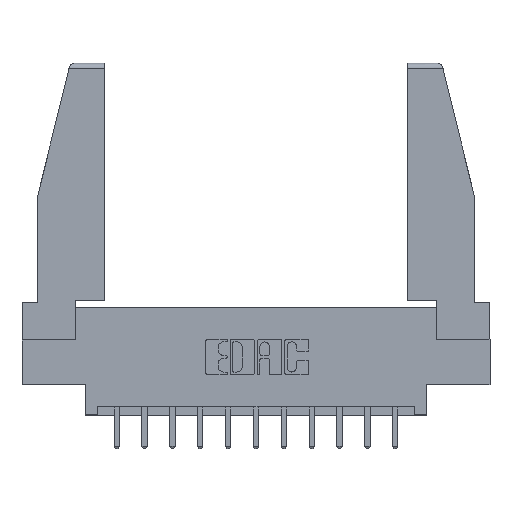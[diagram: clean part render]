
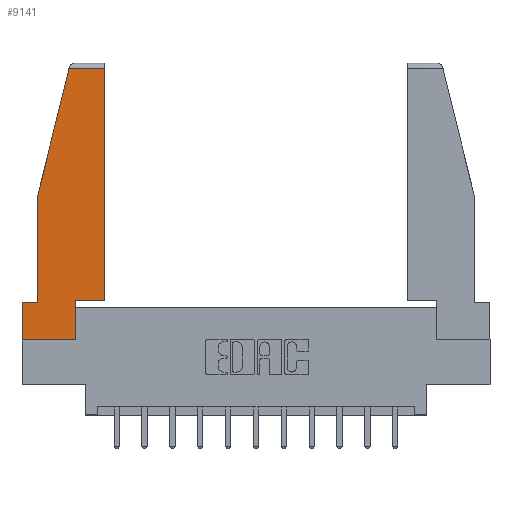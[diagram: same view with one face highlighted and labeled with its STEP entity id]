
A CAD part, top view. The second image highlights one B-rep face of the part: STEP entity #9141.
In plain terms, the highlighted planar face has unit normal (0, 0, 1).
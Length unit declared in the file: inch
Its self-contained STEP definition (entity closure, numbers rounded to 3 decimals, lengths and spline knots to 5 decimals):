
#38 = LINE ( 'NONE', #3504, #4420 ) ;
#55 = CARTESIAN_POINT ( 'NONE',  ( 0.086, 0.21, 0. ) ) ;
#106 = DIRECTION ( 'NONE',  ( 0., -1., 0. ) ) ;
#253 = LINE ( 'NONE', #11143, #9114 ) ;
#321 = LINE ( 'NONE', #2635, #6959 ) ;
#581 = LINE ( 'NONE', #10545, #7043 ) ;
#944 = CARTESIAN_POINT ( 'NONE',  ( 0.297, 0.223, 0. ) ) ;
#1644 = VECTOR ( 'NONE', #15163, 39.37008 ) ;
#1732 = LINE ( 'NONE', #8029, #3739 ) ;
#1884 = DIRECTION ( 'NONE',  ( 1., 0., 0. ) ) ;
#1932 = CARTESIAN_POINT ( 'NONE',  ( 0.086, 0.8, 0. ) ) ;
#1956 = ORIENTED_EDGE ( 'NONE', *, *, #14756, .T. ) ;
#2014 = VERTEX_POINT ( 'NONE', #13711 ) ;
#2033 = EDGE_CURVE ( 'NONE', #5828, #14342, #1732, .T. ) ;
#2052 = ORIENTED_EDGE ( 'NONE', *, *, #15038, .T. ) ;
#2635 = CARTESIAN_POINT ( 'NONE',  ( 0.271, 1.55, 0. ) ) ;
#2669 = EDGE_CURVE ( 'NONE', #5013, #2014, #13351, .T. ) ;
#2760 = VERTEX_POINT ( 'NONE', #4423 ) ;
#3504 = CARTESIAN_POINT ( 'NONE',  ( 0.086, 0.8, 0. ) ) ;
#3529 = VECTOR ( 'NONE', #14760, 39.37008 ) ;
#3739 = VECTOR ( 'NONE', #10301, 39.37008 ) ;
#4176 = ORIENTED_EDGE ( 'NONE', *, *, #2033, .T. ) ;
#4420 = VECTOR ( 'NONE', #106, 39.37008 ) ;
#4423 = CARTESIAN_POINT ( 'NONE',  ( 0.461, 0.223, 0. ) ) ;
#4565 = VECTOR ( 'NONE', #7391, 39.37008 ) ;
#4685 = CARTESIAN_POINT ( 'NONE',  ( 0., 0., 0. ) ) ;
#4693 = DIRECTION ( 'NONE',  ( 1., 0., 0. ) ) ;
#4788 = EDGE_LOOP ( 'NONE', ( #13145, #8458, #7961, #2052, #1956, #14814, #6717, #4176, #9904 ) ) ;
#4796 = CARTESIAN_POINT ( 'NONE',  ( 0., 0., 0. ) ) ;
#5013 = VERTEX_POINT ( 'NONE', #12479 ) ;
#5036 = EDGE_CURVE ( 'NONE', #2760, #5013, #253, .T. ) ;
#5158 = LINE ( 'NONE', #13954, #1644 ) ;
#5407 = PLANE ( 'NONE',  #12798 ) ;
#5488 = CARTESIAN_POINT ( 'NONE',  ( 0., 1.52, 0. ) ) ;
#5490 = FACE_OUTER_BOUND ( 'NONE', #4788, .T. ) ;
#5828 = VERTEX_POINT ( 'NONE', #9521 ) ;
#6447 = DIRECTION ( 'NONE',  ( 0., 1., 0. ) ) ;
#6717 = ORIENTED_EDGE ( 'NONE', *, *, #12679, .T. ) ;
#6959 = VECTOR ( 'NONE', #12005, 39.37008 ) ;
#7043 = VECTOR ( 'NONE', #12926, 39.37008 ) ;
#7085 = VERTEX_POINT ( 'NONE', #4685 ) ;
#7391 = DIRECTION ( 'NONE',  ( 0., -1., 0. ) ) ;
#7961 = ORIENTED_EDGE ( 'NONE', *, *, #9427, .T. ) ;
#8029 = CARTESIAN_POINT ( 'NONE',  ( 0.297, 0., 0. ) ) ;
#8458 = ORIENTED_EDGE ( 'NONE', *, *, #2669, .T. ) ;
#8741 = CARTESIAN_POINT ( 'NONE',  ( 0., 0.21, 0. ) ) ;
#9114 = VECTOR ( 'NONE', #6447, 39.37008 ) ;
#9141 = ADVANCED_FACE ( 'NONE', ( #5490 ), #5407, .T. ) ;
#9427 = EDGE_CURVE ( 'NONE', #2014, #13425, #321, .T. ) ;
#9521 = CARTESIAN_POINT ( 'NONE',  ( 0.297, 0., 0. ) ) ;
#9904 = ORIENTED_EDGE ( 'NONE', *, *, #11215, .T. ) ;
#10243 = VERTEX_POINT ( 'NONE', #55 ) ;
#10301 = DIRECTION ( 'NONE',  ( 0., 1., 0. ) ) ;
#10310 = LINE ( 'NONE', #8741, #4565 ) ;
#10482 = EDGE_CURVE ( 'NONE', #11656, #7085, #10310, .T. ) ;
#10545 = CARTESIAN_POINT ( 'NONE',  ( 0., 0.21, 0. ) ) ;
#10654 = LINE ( 'NONE', #4796, #12468 ) ;
#11143 = CARTESIAN_POINT ( 'NONE',  ( 0.461, 0.223, 0. ) ) ;
#11215 = EDGE_CURVE ( 'NONE', #14342, #2760, #5158, .T. ) ;
#11617 = CARTESIAN_POINT ( 'NONE',  ( 0., 0.21, 0. ) ) ;
#11656 = VERTEX_POINT ( 'NONE', #11617 ) ;
#12005 = DIRECTION ( 'NONE',  ( -0.239, -0.971, 0. ) ) ;
#12468 = VECTOR ( 'NONE', #4693, 39.37008 ) ;
#12479 = CARTESIAN_POINT ( 'NONE',  ( 0.461, 1.52, 0. ) ) ;
#12679 = EDGE_CURVE ( 'NONE', #7085, #5828, #10654, .T. ) ;
#12798 = AXIS2_PLACEMENT_3D ( 'NONE', #13570, #14735, #1884 ) ;
#12926 = DIRECTION ( 'NONE',  ( -1., 0., 0. ) ) ;
#13145 = ORIENTED_EDGE ( 'NONE', *, *, #5036, .T. ) ;
#13351 = LINE ( 'NONE', #5488, #3529 ) ;
#13425 = VERTEX_POINT ( 'NONE', #1932 ) ;
#13570 = CARTESIAN_POINT ( 'NONE',  ( 0., 0., 0. ) ) ;
#13711 = CARTESIAN_POINT ( 'NONE',  ( 0.2636, 1.52, 0. ) ) ;
#13954 = CARTESIAN_POINT ( 'NONE',  ( 0.297, 0.223, 0. ) ) ;
#14342 = VERTEX_POINT ( 'NONE', #944 ) ;
#14735 = DIRECTION ( 'NONE',  ( 0., 0., 1. ) ) ;
#14756 = EDGE_CURVE ( 'NONE', #10243, #11656, #581, .T. ) ;
#14760 = DIRECTION ( 'NONE',  ( -1., 0., 0. ) ) ;
#14814 = ORIENTED_EDGE ( 'NONE', *, *, #10482, .T. ) ;
#15038 = EDGE_CURVE ( 'NONE', #13425, #10243, #38, .T. ) ;
#15163 = DIRECTION ( 'NONE',  ( 1., 0., 0. ) ) ;
